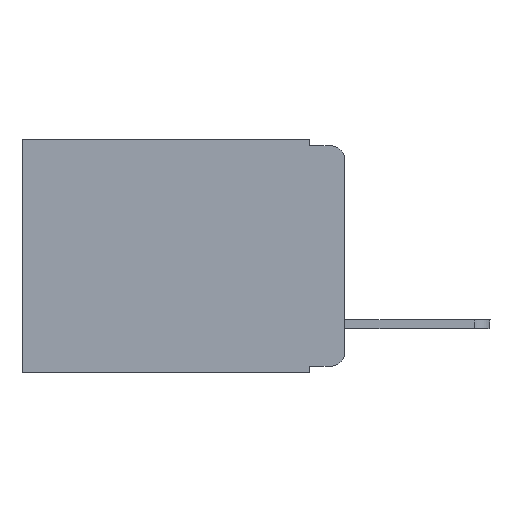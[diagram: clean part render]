
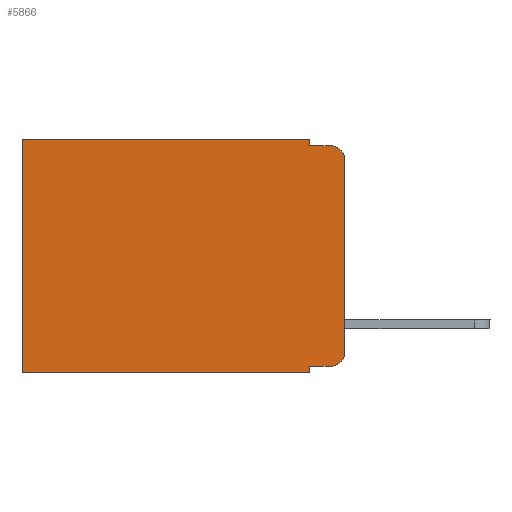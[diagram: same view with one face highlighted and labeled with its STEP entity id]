
A CAD part, left-side view. The second image highlights one B-rep face of the part: STEP entity #5866.
In plain terms, the highlighted planar face has unit normal (-1, 0, 0).
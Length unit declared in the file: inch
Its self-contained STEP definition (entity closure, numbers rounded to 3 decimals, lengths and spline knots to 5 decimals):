
#230 = DIRECTION ( 'NONE',  ( 0., 0., -1. ) ) ;
#683 = EDGE_CURVE ( 'NONE', #4693, #5606, #12066, .T. ) ;
#965 = ORIENTED_EDGE ( 'NONE', *, *, #14290, .F. ) ;
#1080 = DIRECTION ( 'NONE',  ( -1., 0., 0. ) ) ;
#1147 = CARTESIAN_POINT ( 'NONE',  ( 0.298, 0.02, -0.313 ) ) ;
#1268 = VERTEX_POINT ( 'NONE', #16856 ) ;
#2616 = VECTOR ( 'NONE', #19387, 39.37008 ) ;
#2925 = EDGE_CURVE ( 'NONE', #5534, #1268, #13565, .T. ) ;
#3057 = CARTESIAN_POINT ( 'NONE',  ( 0.298, 0.051, -0.333 ) ) ;
#3096 = DIRECTION ( 'NONE',  ( 0., 0., -1. ) ) ;
#3190 = DIRECTION ( 'NONE',  ( 0., 0., -1. ) ) ;
#3479 = DIRECTION ( 'NONE',  ( 1., 0., 0. ) ) ;
#3639 = CARTESIAN_POINT ( 'NONE',  ( 0.298, 0., 0. ) ) ;
#4489 = ORIENTED_EDGE ( 'NONE', *, *, #13821, .T. ) ;
#4693 = VERTEX_POINT ( 'NONE', #4701 ) ;
#4701 = CARTESIAN_POINT ( 'NONE',  ( 0.298, 0., -0.03 ) ) ;
#4855 = CARTESIAN_POINT ( 'NONE',  ( 0.298, 0.02, -0.01 ) ) ;
#4938 = EDGE_CURVE ( 'NONE', #11953, #5606, #20234, .T. ) ;
#5507 = DIRECTION ( 'NONE',  ( 0., 1., 0. ) ) ;
#5521 = EDGE_CURVE ( 'NONE', #15764, #11953, #16028, .T. ) ;
#5534 = VERTEX_POINT ( 'NONE', #3057 ) ;
#5606 = VERTEX_POINT ( 'NONE', #4855 ) ;
#5866 = ADVANCED_FACE ( 'NONE', ( #18019 ), #8218, .F. ) ;
#5895 = AXIS2_PLACEMENT_3D ( 'NONE', #8700, #12249, #17140 ) ;
#6179 = DIRECTION ( 'NONE',  ( 0., 0., -1. ) ) ;
#6180 = DIRECTION ( 'NONE',  ( 0., -1., 0. ) ) ;
#6405 = VECTOR ( 'NONE', #5507, 39.37008 ) ;
#6498 = AXIS2_PLACEMENT_3D ( 'NONE', #3639, #3479, #230 ) ;
#6769 = ORIENTED_EDGE ( 'NONE', *, *, #5521, .F. ) ;
#6808 = EDGE_CURVE ( 'NONE', #1268, #13619, #11078, .T. ) ;
#6835 = LINE ( 'NONE', #19170, #10511 ) ;
#7281 = CARTESIAN_POINT ( 'NONE',  ( 0.298, 0., 0. ) ) ;
#7881 = VERTEX_POINT ( 'NONE', #8869 ) ;
#7947 = VECTOR ( 'NONE', #3190, 39.37008 ) ;
#8218 = PLANE ( 'NONE',  #6498 ) ;
#8300 = EDGE_CURVE ( 'NONE', #18918, #13619, #6835, .T. ) ;
#8355 = CARTESIAN_POINT ( 'NONE',  ( 0.298, 0.051, 0. ) ) ;
#8417 = CARTESIAN_POINT ( 'NONE',  ( 0.298, 0.473, 0. ) ) ;
#8700 = CARTESIAN_POINT ( 'NONE',  ( 0.298, 0.02, -0.03 ) ) ;
#8869 = CARTESIAN_POINT ( 'NONE',  ( 0.298, 0., -0.313 ) ) ;
#8881 = DIRECTION ( 'NONE',  ( 0., 0., -1. ) ) ;
#9273 = CIRCLE ( 'NONE', #15948, 0.02 ) ;
#9515 = CARTESIAN_POINT ( 'NONE',  ( 0.298, 0.473, -0.343 ) ) ;
#9628 = ORIENTED_EDGE ( 'NONE', *, *, #8300, .T. ) ;
#10020 = ORIENTED_EDGE ( 'NONE', *, *, #2925, .F. ) ;
#10109 = VECTOR ( 'NONE', #10141, 39.37008 ) ;
#10141 = DIRECTION ( 'NONE',  ( 0., 1., 0. ) ) ;
#10511 = VECTOR ( 'NONE', #14564, 39.37008 ) ;
#10522 = ORIENTED_EDGE ( 'NONE', *, *, #6808, .F. ) ;
#10578 = LINE ( 'NONE', #7281, #6405 ) ;
#11067 = EDGE_LOOP ( 'NONE', ( #965, #14188, #17794, #6769, #4489, #9628, #10522, #10020, #18340, #20161 ) ) ;
#11078 = LINE ( 'NONE', #14800, #10109 ) ;
#11455 = VECTOR ( 'NONE', #6180, 39.37008 ) ;
#11953 = VERTEX_POINT ( 'NONE', #13890 ) ;
#12009 = LINE ( 'NONE', #13845, #13706 ) ;
#12066 = CIRCLE ( 'NONE', #5895, 0.02 ) ;
#12249 = DIRECTION ( 'NONE',  ( -1., 0., 0. ) ) ;
#12400 = CARTESIAN_POINT ( 'NONE',  ( 0.298, 0.051, -0.333 ) ) ;
#13059 = VECTOR ( 'NONE', #6179, 39.37008 ) ;
#13565 = LINE ( 'NONE', #18878, #13059 ) ;
#13619 = VERTEX_POINT ( 'NONE', #9515 ) ;
#13706 = VECTOR ( 'NONE', #3096, 39.37008 ) ;
#13821 = EDGE_CURVE ( 'NONE', #15764, #18918, #10578, .T. ) ;
#13845 = CARTESIAN_POINT ( 'NONE',  ( 0.298, 0., 0. ) ) ;
#13890 = CARTESIAN_POINT ( 'NONE',  ( 0.298, 0.051, -0.01 ) ) ;
#14188 = ORIENTED_EDGE ( 'NONE', *, *, #683, .T. ) ;
#14290 = EDGE_CURVE ( 'NONE', #4693, #7881, #12009, .T. ) ;
#14564 = DIRECTION ( 'NONE',  ( 0., 0., -1. ) ) ;
#14783 = CARTESIAN_POINT ( 'NONE',  ( 0.298, 0.051, -0.01 ) ) ;
#14800 = CARTESIAN_POINT ( 'NONE',  ( 0.298, 0., -0.343 ) ) ;
#15383 = EDGE_CURVE ( 'NONE', #18987, #7881, #9273, .T. ) ;
#15618 = LINE ( 'NONE', #12400, #11455 ) ;
#15764 = VERTEX_POINT ( 'NONE', #8355 ) ;
#15948 = AXIS2_PLACEMENT_3D ( 'NONE', #1147, #1080, #8881 ) ;
#16028 = LINE ( 'NONE', #18904, #7947 ) ;
#16602 = EDGE_CURVE ( 'NONE', #5534, #18987, #15618, .T. ) ;
#16856 = CARTESIAN_POINT ( 'NONE',  ( 0.298, 0.051, -0.343 ) ) ;
#17140 = DIRECTION ( 'NONE',  ( 0., 0., -1. ) ) ;
#17794 = ORIENTED_EDGE ( 'NONE', *, *, #4938, .F. ) ;
#18019 = FACE_OUTER_BOUND ( 'NONE', #11067, .T. ) ;
#18235 = CARTESIAN_POINT ( 'NONE',  ( 0.298, 0.02, -0.333 ) ) ;
#18340 = ORIENTED_EDGE ( 'NONE', *, *, #16602, .T. ) ;
#18878 = CARTESIAN_POINT ( 'NONE',  ( 0.298, 0.051, 0. ) ) ;
#18904 = CARTESIAN_POINT ( 'NONE',  ( 0.298, 0.051, 0. ) ) ;
#18918 = VERTEX_POINT ( 'NONE', #8417 ) ;
#18987 = VERTEX_POINT ( 'NONE', #18235 ) ;
#19170 = CARTESIAN_POINT ( 'NONE',  ( 0.298, 0.473, 0. ) ) ;
#19387 = DIRECTION ( 'NONE',  ( 0., -1., 0. ) ) ;
#20161 = ORIENTED_EDGE ( 'NONE', *, *, #15383, .T. ) ;
#20234 = LINE ( 'NONE', #14783, #2616 ) ;
